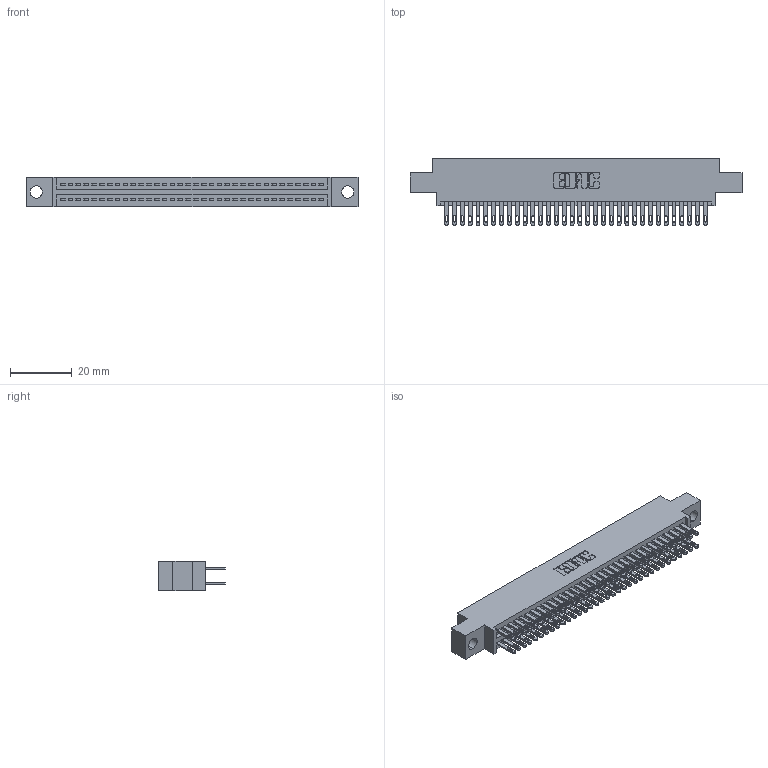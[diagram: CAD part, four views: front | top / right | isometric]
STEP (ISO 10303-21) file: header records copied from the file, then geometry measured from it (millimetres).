
FILE_DESCRIPTION (( 'STEP AP203' ), '1' );
FILE_NAME ('345-068-500-804.STEP', '2021-05-20T07:31:58', ( '' ), ( '' ), 'SwSTEP 2.0', 'SolidWorks 2020', '' );
FILE_SCHEMA (( 'CONFIG_CONTROL_DESIGN' ));
Length unit declared in the file: inch
Products named in the file (3): 345 Part_0.170 Offset - 0.156 Dia-TI; 345-068-500-804; 345-292-001_345-293-100
Assembly tree (69 placements, depth 2):
  345-068-500-804
    345 Part_0.170 Offset - 0.156 Dia-TI
    345-292-001_345-293-100  x68
Bounding box: 107.57 x 21.51 x 9.4 mm (x, y, z)
Volume: 10363.6 mm3; surface area: 15852.8 mm2
Topology: 69 solids, 69 shells, 3272 faces, 9977 edges, 6650 vertices
Faces by surface type: plane 1934, cylinder 1338
Entity records: 28235 total; most frequent: CARTESIAN_POINT 4746, ORIENTED_EDGE 4678, DIRECTION 4195, EDGE_CURVE 2339, LINE 2067, VECTOR 2067, VERTEX_POINT 1558, AXIS2_PLACEMENT_3D 1064
